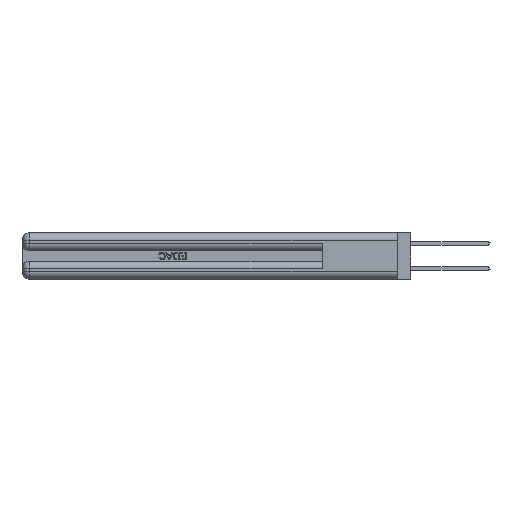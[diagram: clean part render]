
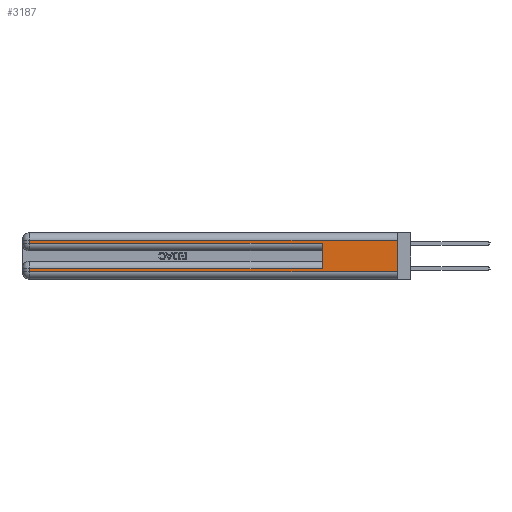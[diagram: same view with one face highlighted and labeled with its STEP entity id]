
A CAD part, left-side view. The second image highlights one B-rep face of the part: STEP entity #3187.
In plain terms, the highlighted planar face has unit normal (-1, 0, 0).
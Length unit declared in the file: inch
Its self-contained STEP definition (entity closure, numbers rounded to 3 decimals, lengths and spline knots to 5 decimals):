
#348 = DIRECTION ( 'NONE',  ( 1., 0., 0. ) ) ;
#391 = DIRECTION ( 'NONE',  ( 0., 0., -1. ) ) ;
#598 = VERTEX_POINT ( 'NONE', #3929 ) ;
#755 = CARTESIAN_POINT ( 'NONE',  ( 0., 2.94, 0.37 ) ) ;
#795 = CARTESIAN_POINT ( 'NONE',  ( 0., 2.94, 0.085 ) ) ;
#1630 = ORIENTED_EDGE ( 'NONE', *, *, #26583, .T. ) ;
#1789 = FACE_OUTER_BOUND ( 'NONE', #43270, .T. ) ;
#3187 = ADVANCED_FACE ( 'NONE', ( #1789 ), #23681, .F. ) ;
#3293 = VECTOR ( 'NONE', #26257, 39.37008 ) ;
#3929 = CARTESIAN_POINT ( 'NONE',  ( 0., 2.94, 0.06 ) ) ;
#5264 = ORIENTED_EDGE ( 'NONE', *, *, #44959, .T. ) ;
#6091 = LINE ( 'NONE', #27448, #35778 ) ;
#6424 = EDGE_CURVE ( 'NONE', #22601, #598, #40615, .T. ) ;
#6496 = EDGE_CURVE ( 'NONE', #46925, #33858, #6091, .T. ) ;
#6682 = CARTESIAN_POINT ( 'NONE',  ( 0., 0.6, 0.285 ) ) ;
#6870 = VECTOR ( 'NONE', #9645, 39.37008 ) ;
#6973 = CARTESIAN_POINT ( 'NONE',  ( 0., 0., 0.06 ) ) ;
#7675 = CARTESIAN_POINT ( 'NONE',  ( 0., 2.94, 0.37 ) ) ;
#8483 = CARTESIAN_POINT ( 'NONE',  ( 0., 0., 0.085 ) ) ;
#8550 = VECTOR ( 'NONE', #46306, 39.37008 ) ;
#8944 = ORIENTED_EDGE ( 'NONE', *, *, #48420, .T. ) ;
#9645 = DIRECTION ( 'NONE',  ( 0., 0., 1. ) ) ;
#12365 = DIRECTION ( 'NONE',  ( 0., 1., 0. ) ) ;
#14361 = VECTOR ( 'NONE', #46244, 39.37008 ) ;
#15389 = CARTESIAN_POINT ( 'NONE',  ( 0., 0., 0.31 ) ) ;
#15553 = EDGE_CURVE ( 'NONE', #42192, #49751, #36547, .T. ) ;
#16804 = LINE ( 'NONE', #15389, #14361 ) ;
#17285 = DIRECTION ( 'NONE',  ( 0., -1., 0. ) ) ;
#20820 = CARTESIAN_POINT ( 'NONE',  ( 0., 2.94, 0.285 ) ) ;
#21118 = CARTESIAN_POINT ( 'NONE',  ( 0., 0.6, 0.145 ) ) ;
#21168 = CARTESIAN_POINT ( 'NONE',  ( 0., 0., 0.31 ) ) ;
#22601 = VERTEX_POINT ( 'NONE', #795 ) ;
#23681 = PLANE ( 'NONE',  #38903 ) ;
#24632 = ORIENTED_EDGE ( 'NONE', *, *, #35353, .T. ) ;
#24879 = CARTESIAN_POINT ( 'NONE',  ( 0., 0., 0.285 ) ) ;
#24955 = LINE ( 'NONE', #24879, #38880 ) ;
#26257 = DIRECTION ( 'NONE',  ( 0., -1., 0. ) ) ;
#26583 = EDGE_CURVE ( 'NONE', #43849, #48841, #39571, .T. ) ;
#27448 = CARTESIAN_POINT ( 'NONE',  ( 0., 0., 0.37 ) ) ;
#27580 = DIRECTION ( 'NONE',  ( 0., 0., -1. ) ) ;
#27823 = DIRECTION ( 'NONE',  ( 0., 0., -1. ) ) ;
#28291 = ORIENTED_EDGE ( 'NONE', *, *, #6424, .T. ) ;
#28478 = LINE ( 'NONE', #8483, #47748 ) ;
#29297 = VECTOR ( 'NONE', #27823, 39.37008 ) ;
#29377 = CARTESIAN_POINT ( 'NONE',  ( 0., 2.94, 0.31 ) ) ;
#29847 = CARTESIAN_POINT ( 'NONE',  ( 0., 0.6, 0.085 ) ) ;
#31296 = ORIENTED_EDGE ( 'NONE', *, *, #47249, .T. ) ;
#33858 = VERTEX_POINT ( 'NONE', #39902 ) ;
#34216 = LINE ( 'NONE', #6973, #3293 ) ;
#34935 = ORIENTED_EDGE ( 'NONE', *, *, #15553, .F. ) ;
#35353 = EDGE_CURVE ( 'NONE', #48841, #49751, #24955, .T. ) ;
#35778 = VECTOR ( 'NONE', #391, 39.37008 ) ;
#36547 = LINE ( 'NONE', #21118, #6870 ) ;
#37933 = ORIENTED_EDGE ( 'NONE', *, *, #6496, .F. ) ;
#38880 = VECTOR ( 'NONE', #17285, 39.37008 ) ;
#38903 = AXIS2_PLACEMENT_3D ( 'NONE', #42905, #348, #27580 ) ;
#39571 = LINE ( 'NONE', #755, #29297 ) ;
#39902 = CARTESIAN_POINT ( 'NONE',  ( 0., 0., 0.06 ) ) ;
#40615 = LINE ( 'NONE', #7675, #8550 ) ;
#42192 = VERTEX_POINT ( 'NONE', #29847 ) ;
#42905 = CARTESIAN_POINT ( 'NONE',  ( 0., 0., 0.37 ) ) ;
#43270 = EDGE_LOOP ( 'NONE', ( #37933, #31296, #1630, #24632, #34935, #5264, #28291, #8944 ) ) ;
#43849 = VERTEX_POINT ( 'NONE', #29377 ) ;
#44959 = EDGE_CURVE ( 'NONE', #42192, #22601, #28478, .T. ) ;
#46244 = DIRECTION ( 'NONE',  ( 0., 1., 0. ) ) ;
#46306 = DIRECTION ( 'NONE',  ( 0., 0., -1. ) ) ;
#46925 = VERTEX_POINT ( 'NONE', #21168 ) ;
#47249 = EDGE_CURVE ( 'NONE', #46925, #43849, #16804, .T. ) ;
#47748 = VECTOR ( 'NONE', #12365, 39.37008 ) ;
#48420 = EDGE_CURVE ( 'NONE', #598, #33858, #34216, .T. ) ;
#48841 = VERTEX_POINT ( 'NONE', #20820 ) ;
#49751 = VERTEX_POINT ( 'NONE', #6682 ) ;
